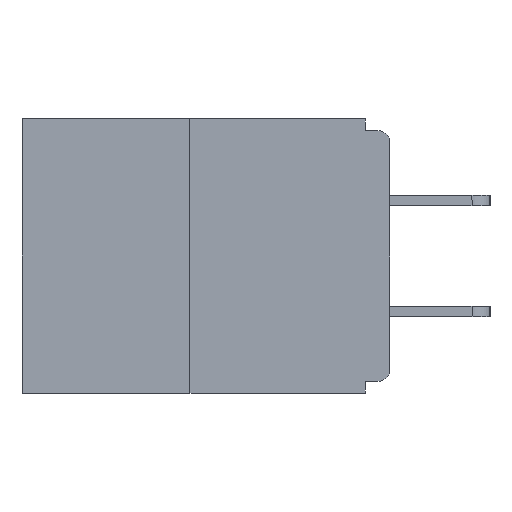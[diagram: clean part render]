
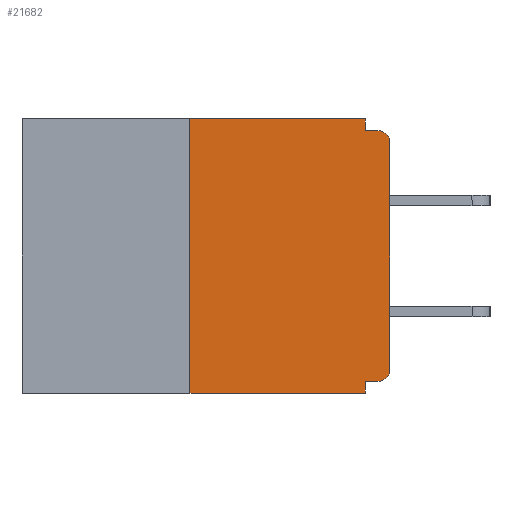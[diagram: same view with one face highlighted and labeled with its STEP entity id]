
A CAD part, left-side view. The second image highlights one B-rep face of the part: STEP entity #21682.
In plain terms, the highlighted planar face has unit normal (-1, 0, 0).
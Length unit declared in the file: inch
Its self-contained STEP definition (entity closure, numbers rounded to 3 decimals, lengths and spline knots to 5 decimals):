
#1 = CARTESIAN_POINT ( 'NONE',  ( 0., 0.031, -0.015 ) ) ;
#108 = LINE ( 'NONE', #12269, #3979 ) ;
#421 = CARTESIAN_POINT ( 'NONE',  ( 0., 0., 0. ) ) ;
#576 = EDGE_CURVE ( 'NONE', #6105, #22155, #21223, .T. ) ;
#605 = VERTEX_POINT ( 'NONE', #24111 ) ;
#770 = AXIS2_PLACEMENT_3D ( 'NONE', #17248, #11712, #22856 ) ;
#980 = PLANE ( 'NONE',  #17133 ) ;
#1222 = EDGE_CURVE ( 'NONE', #18066, #27560, #17049, .T. ) ;
#1590 = ORIENTED_EDGE ( 'NONE', *, *, #14582, .F. ) ;
#2979 = VECTOR ( 'NONE', #20667, 39.37008 ) ;
#3230 = ORIENTED_EDGE ( 'NONE', *, *, #25335, .T. ) ;
#3246 = CARTESIAN_POINT ( 'NONE',  ( 0., 0., -0.03 ) ) ;
#3979 = VECTOR ( 'NONE', #27677, 39.37008 ) ;
#5839 = CARTESIAN_POINT ( 'NONE',  ( 0., 0.25, 0. ) ) ;
#6105 = VERTEX_POINT ( 'NONE', #5839 ) ;
#6161 = DIRECTION ( 'NONE',  ( 0., -1., 0. ) ) ;
#6352 = CIRCLE ( 'NONE', #770, 0.015 ) ;
#6794 = VECTOR ( 'NONE', #6161, 39.37008 ) ;
#7247 = CARTESIAN_POINT ( 'NONE',  ( 0., 0.031, -0.343 ) ) ;
#7682 = VECTOR ( 'NONE', #9316, 39.37008 ) ;
#7727 = EDGE_CURVE ( 'NONE', #27152, #27560, #6352, .T. ) ;
#8498 = ORIENTED_EDGE ( 'NONE', *, *, #20158, .F. ) ;
#8522 = CARTESIAN_POINT ( 'NONE',  ( 0., 0.015, -0.328 ) ) ;
#8849 = CARTESIAN_POINT ( 'NONE',  ( 0., 0.25, 0. ) ) ;
#9316 = DIRECTION ( 'NONE',  ( 0., 0., 1. ) ) ;
#10235 = EDGE_CURVE ( 'NONE', #25510, #14773, #18145, .T. ) ;
#10530 = CARTESIAN_POINT ( 'NONE',  ( 0., 0.46, 0. ) ) ;
#10760 = ORIENTED_EDGE ( 'NONE', *, *, #18127, .F. ) ;
#11117 = ORIENTED_EDGE ( 'NONE', *, *, #14028, .F. ) ;
#11712 = DIRECTION ( 'NONE',  ( -1., 0., 0. ) ) ;
#12269 = CARTESIAN_POINT ( 'NONE',  ( 0., 0.46, -0.343 ) ) ;
#12985 = ORIENTED_EDGE ( 'NONE', *, *, #7727, .T. ) ;
#13512 = ORIENTED_EDGE ( 'NONE', *, *, #1222, .F. ) ;
#13531 = CARTESIAN_POINT ( 'NONE',  ( 0., 0., -0.313 ) ) ;
#13543 = ORIENTED_EDGE ( 'NONE', *, *, #576, .F. ) ;
#13642 = EDGE_CURVE ( 'NONE', #14773, #27152, #13868, .T. ) ;
#13835 = LINE ( 'NONE', #7247, #24814 ) ;
#13863 = DIRECTION ( 'NONE',  ( 0., 0., -1. ) ) ;
#13868 = LINE ( 'NONE', #421, #7682 ) ;
#14028 = EDGE_CURVE ( 'NONE', #20353, #24923, #13835, .T. ) ;
#14229 = DIRECTION ( 'NONE',  ( 0., -1., 0. ) ) ;
#14582 = EDGE_CURVE ( 'NONE', #22155, #18066, #15795, .T. ) ;
#14773 = VERTEX_POINT ( 'NONE', #13531 ) ;
#14952 = CARTESIAN_POINT ( 'NONE',  ( 0., 0.015, -0.015 ) ) ;
#15105 = FACE_OUTER_BOUND ( 'NONE', #21349, .T. ) ;
#15285 = LINE ( 'NONE', #16120, #2979 ) ;
#15795 = LINE ( 'NONE', #23613, #16854 ) ;
#16120 = CARTESIAN_POINT ( 'NONE',  ( 0., 0., -0.328 ) ) ;
#16854 = VECTOR ( 'NONE', #25625, 39.37008 ) ;
#16993 = DIRECTION ( 'NONE',  ( 1., 0., 0. ) ) ;
#17049 = LINE ( 'NONE', #17161, #6794 ) ;
#17133 = AXIS2_PLACEMENT_3D ( 'NONE', #10530, #16993, #23446 ) ;
#17161 = CARTESIAN_POINT ( 'NONE',  ( 0., 0., -0.015 ) ) ;
#17248 = CARTESIAN_POINT ( 'NONE',  ( 0., 0.015, -0.03 ) ) ;
#17451 = ORIENTED_EDGE ( 'NONE', *, *, #10235, .T. ) ;
#17697 = CARTESIAN_POINT ( 'NONE',  ( 0., 0.015, -0.313 ) ) ;
#18066 = VERTEX_POINT ( 'NONE', #1 ) ;
#18127 = EDGE_CURVE ( 'NONE', #25510, #20353, #15285, .T. ) ;
#18145 = CIRCLE ( 'NONE', #23081, 0.015 ) ;
#18595 = LINE ( 'NONE', #8849, #20313 ) ;
#18676 = CARTESIAN_POINT ( 'NONE',  ( 0., 0.031, -0.328 ) ) ;
#19734 = CARTESIAN_POINT ( 'NONE',  ( 0., 0.031, -0.343 ) ) ;
#20158 = EDGE_CURVE ( 'NONE', #605, #6105, #18595, .T. ) ;
#20313 = VECTOR ( 'NONE', #28116, 39.37008 ) ;
#20353 = VERTEX_POINT ( 'NONE', #18676 ) ;
#20667 = DIRECTION ( 'NONE',  ( 0., 1., 0. ) ) ;
#21223 = LINE ( 'NONE', #22164, #22616 ) ;
#21349 = EDGE_LOOP ( 'NONE', ( #13543, #8498, #3230, #11117, #10760, #17451, #22405, #12985, #13512, #1590 ) ) ;
#21682 = ADVANCED_FACE ( 'NONE', ( #15105 ), #980, .F. ) ;
#21734 = DIRECTION ( 'NONE',  ( 0., 0., -1. ) ) ;
#22155 = VERTEX_POINT ( 'NONE', #23799 ) ;
#22164 = CARTESIAN_POINT ( 'NONE',  ( 0., 0.46, 0. ) ) ;
#22405 = ORIENTED_EDGE ( 'NONE', *, *, #13642, .T. ) ;
#22616 = VECTOR ( 'NONE', #14229, 39.37008 ) ;
#22856 = DIRECTION ( 'NONE',  ( 0., 0., -1. ) ) ;
#23081 = AXIS2_PLACEMENT_3D ( 'NONE', #17697, #26254, #21734 ) ;
#23446 = DIRECTION ( 'NONE',  ( 0., 0., -1. ) ) ;
#23613 = CARTESIAN_POINT ( 'NONE',  ( 0., 0.031, 0. ) ) ;
#23799 = CARTESIAN_POINT ( 'NONE',  ( 0., 0.031, 0. ) ) ;
#24111 = CARTESIAN_POINT ( 'NONE',  ( 0., 0.25, -0.343 ) ) ;
#24814 = VECTOR ( 'NONE', #13863, 39.37008 ) ;
#24923 = VERTEX_POINT ( 'NONE', #19734 ) ;
#25335 = EDGE_CURVE ( 'NONE', #605, #24923, #108, .T. ) ;
#25510 = VERTEX_POINT ( 'NONE', #8522 ) ;
#25625 = DIRECTION ( 'NONE',  ( 0., 0., -1. ) ) ;
#26254 = DIRECTION ( 'NONE',  ( -1., 0., 0. ) ) ;
#27152 = VERTEX_POINT ( 'NONE', #3246 ) ;
#27560 = VERTEX_POINT ( 'NONE', #14952 ) ;
#27677 = DIRECTION ( 'NONE',  ( 0., -1., 0. ) ) ;
#28116 = DIRECTION ( 'NONE',  ( 0., 0., 1. ) ) ;
